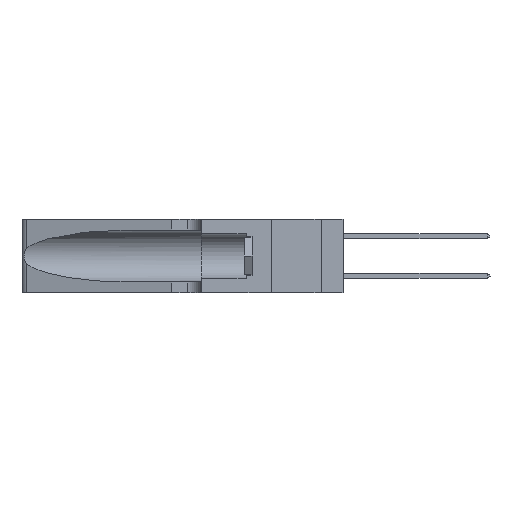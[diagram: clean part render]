
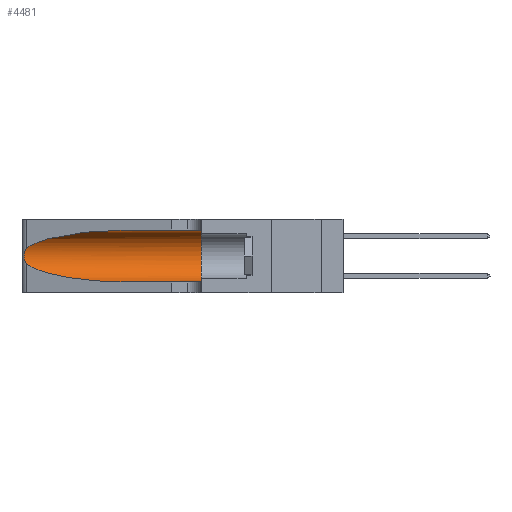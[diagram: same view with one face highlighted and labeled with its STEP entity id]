
A CAD part, left-side view. The second image highlights one B-rep face of the part: STEP entity #4481.
In plain terms, the highlighted cylindrical face has radius 3.308 mm (diameter 6.617 mm), a partial arc.
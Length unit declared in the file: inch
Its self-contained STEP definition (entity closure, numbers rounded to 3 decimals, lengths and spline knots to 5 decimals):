
#8 = CARTESIAN_POINT ( 'NONE',  ( 0.1305, 0.35, 0.05475 ) ) ;
#198 = AXIS2_PLACEMENT_3D ( 'NONE', #5121, #9780, #26743 ) ;
#911 = CIRCLE ( 'NONE', #198, 0.13025 ) ;
#1108 = VECTOR ( 'NONE', #10877, 39.37008 ) ;
#1569 = CARTESIAN_POINT ( 'NONE',  ( 0.25487, 1.22718, 0.14631 ) ) ;
#2969 = CARTESIAN_POINT ( 'NONE',  ( 0.25854, 1.2359, 0.20912 ) ) ;
#3581 = CARTESIAN_POINT ( 'NONE',  ( 0.1305, 0.72297, 0.31525 ) ) ;
#4358 = EDGE_CURVE ( 'NONE', #14241, #6584, #7115, .T. ) ;
#4481 = ADVANCED_FACE ( 'NONE', ( #8632 ), #23788, .F. ) ;
#5121 = CARTESIAN_POINT ( 'NONE',  ( 0.1305, 0.35, 0.185 ) ) ;
#5875 = ORIENTED_EDGE ( 'NONE', *, *, #20027, .F. ) ;
#6395 = ORIENTED_EDGE ( 'NONE', *, *, #13589, .T. ) ;
#6479 = CARTESIAN_POINT ( 'NONE',  ( 0.26017, 1.23833, 0.17102 ) ) ;
#6584 = VERTEX_POINT ( 'NONE', #8 ) ;
#6792 = CARTESIAN_POINT ( 'NONE',  ( 0.25555, 1.22993, 0.14849 ) ) ;
#7115 = LINE ( 'NONE', #27726, #1108 ) ;
#7119 = ORIENTED_EDGE ( 'NONE', *, *, #4358, .T. ) ;
#7379 = AXIS2_PLACEMENT_3D ( 'NONE', #19871, #27209, #26472 ) ;
#8489 = VECTOR ( 'NONE', #27441, 39.37008 ) ;
#8632 = FACE_OUTER_BOUND ( 'NONE', #25883, .T. ) ;
#8636 = CARTESIAN_POINT ( 'NONE',  ( 0.18966, 0.96281, 0.31525 ) ) ;
#9055 = VERTEX_POINT ( 'NONE', #26261 ) ;
#9128 = CARTESIAN_POINT ( 'NONE',  ( 0.25856, 1.23593, 0.16098 ) ) ;
#9199 = VERTEX_POINT ( 'NONE', #30344 ) ;
#9281 = CARTESIAN_POINT ( 'NONE',  ( 0.2373, 1.15595, 0.08982 ) ) ;
#9780 = DIRECTION ( 'NONE',  ( 0., 1., 0. ) ) ;
#10573 = EDGE_CURVE ( 'NONE', #22179, #9055, #24012, .T. ) ;
#10877 = DIRECTION ( 'NONE',  ( 0., -1., 0. ) ) ;
#11218 = EDGE_CURVE ( 'NONE', #15581, #14241, #19332, .T. ) ;
#12402 = CARTESIAN_POINT ( 'NONE',  ( 0.26075, 1.23896, 0.19203 ) ) ;
#12516 = ORIENTED_EDGE ( 'NONE', *, *, #10573, .F. ) ;
#13589 = EDGE_CURVE ( 'NONE', #9199, #15581, #23762, .T. ) ;
#14241 = VERTEX_POINT ( 'NONE', #23807 ) ;
#14355 = CARTESIAN_POINT ( 'NONE',  ( 0.25639, 1.23184, 0.21858 ) ) ;
#14645 = CARTESIAN_POINT ( 'NONE',  ( 0.25787, 1.23484, 0.2124 ) ) ;
#15581 = VERTEX_POINT ( 'NONE', #16956 ) ;
#16550 = ORIENTED_EDGE ( 'NONE', *, *, #24076, .T. ) ;
#16639 = CARTESIAN_POINT ( 'NONE',  ( 0.1305, 0.72297, 0.05475 ) ) ;
#16956 = CARTESIAN_POINT ( 'NONE',  ( 0.25487, 1.22718, 0.14631 ) ) ;
#18583 = CARTESIAN_POINT ( 'NONE',  ( 0.1305, 0.72297, 0.31525 ) ) ;
#19332 =( BOUNDED_CURVE ( )  B_SPLINE_CURVE ( 3, ( #31327, #9281, #24066, #16639 ),
 .UNSPECIFIED., .F., .F. ) 
 B_SPLINE_CURVE_WITH_KNOTS ( ( 4, 4 ),
 ( 3.44316, 4.71239 ),
 .UNSPECIFIED. ) 
 CURVE ( )  GEOMETRIC_REPRESENTATION_ITEM ( )  RATIONAL_B_SPLINE_CURVE ( ( 1., 0.87, 0.87, 1. ) ) 
 REPRESENTATION_ITEM ( '' )  );
#19871 = CARTESIAN_POINT ( 'NONE',  ( 0.1305, 1.61858, 0.185 ) ) ;
#20027 = EDGE_CURVE ( 'NONE', #9055, #6584, #911, .T. ) ;
#20640 = CARTESIAN_POINT ( 'NONE',  ( 0.26075, 1.23896, 0.178 ) ) ;
#20683 = CARTESIAN_POINT ( 'NONE',  ( 0.2373, 1.15595, 0.28018 ) ) ;
#22179 = VERTEX_POINT ( 'NONE', #18583 ) ;
#23505 = CARTESIAN_POINT ( 'NONE',  ( 0.25789, 1.23486, 0.15765 ) ) ;
#23762 = B_SPLINE_CURVE_WITH_KNOTS ( 'NONE', 3,
 ( #26386, #23928, #14355, #14645, #2969, #23959, #12402, #20640, #6479, #9128, #23505, #26088, #6792, #1569 ),
 .UNSPECIFIED., .F., .F.,
 ( 4, 2, 2, 2, 2, 2, 4 ),
 ( 0., 0.00027, 0.00053, 0.00107, 0.0016, 0.00187, 0.00214 ),
 .UNSPECIFIED. ) ;
#23788 = CYLINDRICAL_SURFACE ( 'NONE', #7379, 0.13025 ) ;
#23807 = CARTESIAN_POINT ( 'NONE',  ( 0.1305, 0.72297, 0.05475 ) ) ;
#23928 = CARTESIAN_POINT ( 'NONE',  ( 0.25555, 1.22994, 0.2215 ) ) ;
#23959 = CARTESIAN_POINT ( 'NONE',  ( 0.26018, 1.23835, 0.19895 ) ) ;
#24012 = LINE ( 'NONE', #25464, #8489 ) ;
#24066 = CARTESIAN_POINT ( 'NONE',  ( 0.18966, 0.96281, 0.05475 ) ) ;
#24076 = EDGE_CURVE ( 'NONE', #22179, #9199, #25543, .T. ) ;
#25464 = CARTESIAN_POINT ( 'NONE',  ( 0.1305, 1.61858, 0.31525 ) ) ;
#25543 =( BOUNDED_CURVE ( )  B_SPLINE_CURVE ( 3, ( #3581, #8636, #20683, #25702 ),
 .UNSPECIFIED., .F., .F. ) 
 B_SPLINE_CURVE_WITH_KNOTS ( ( 4, 4 ),
 ( 1.5708, 2.84003 ),
 .UNSPECIFIED. ) 
 CURVE ( )  GEOMETRIC_REPRESENTATION_ITEM ( )  RATIONAL_B_SPLINE_CURVE ( ( 1., 0.87, 0.87, 1. ) ) 
 REPRESENTATION_ITEM ( '' )  );
#25702 = CARTESIAN_POINT ( 'NONE',  ( 0.25487, 1.22718, 0.22369 ) ) ;
#25883 = EDGE_LOOP ( 'NONE', ( #16550, #6395, #29643, #7119, #5875, #12516 ) ) ;
#26088 = CARTESIAN_POINT ( 'NONE',  ( 0.25639, 1.23186, 0.15144 ) ) ;
#26261 = CARTESIAN_POINT ( 'NONE',  ( 0.1305, 0.35, 0.31525 ) ) ;
#26386 = CARTESIAN_POINT ( 'NONE',  ( 0.25487, 1.22718, 0.22369 ) ) ;
#26472 = DIRECTION ( 'NONE',  ( 0., 0., -1. ) ) ;
#26743 = DIRECTION ( 'NONE',  ( 0., 0., 1. ) ) ;
#27209 = DIRECTION ( 'NONE',  ( 0., -1., 0. ) ) ;
#27441 = DIRECTION ( 'NONE',  ( 0., -1., 0. ) ) ;
#27726 = CARTESIAN_POINT ( 'NONE',  ( 0.1305, 1.61858, 0.05475 ) ) ;
#29643 = ORIENTED_EDGE ( 'NONE', *, *, #11218, .T. ) ;
#30344 = CARTESIAN_POINT ( 'NONE',  ( 0.25487, 1.22718, 0.22369 ) ) ;
#31327 = CARTESIAN_POINT ( 'NONE',  ( 0.25487, 1.22718, 0.14631 ) ) ;
